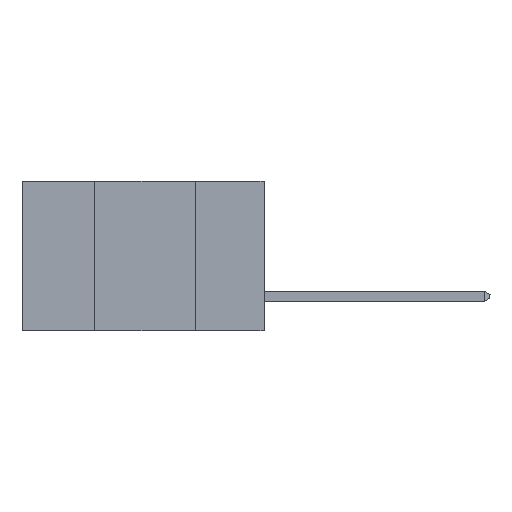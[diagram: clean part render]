
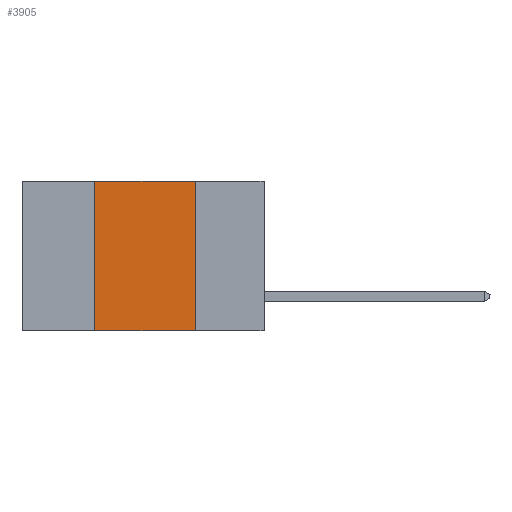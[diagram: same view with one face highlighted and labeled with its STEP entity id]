
A CAD part, left-side view. The second image highlights one B-rep face of the part: STEP entity #3905.
In plain terms, the highlighted planar face has unit normal (-1, 0, 0).
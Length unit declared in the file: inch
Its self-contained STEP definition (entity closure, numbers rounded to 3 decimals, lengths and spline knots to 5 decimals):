
#182 = LINE ( 'NONE', #5513, #4247 ) ;
#1077 = VECTOR ( 'NONE', #8774, 39.37008 ) ;
#1508 = EDGE_CURVE ( 'NONE', #16776, #15488, #14772, .T. ) ;
#1599 = CARTESIAN_POINT ( 'NONE',  ( 0., 0.17, -0.37 ) ) ;
#1852 = VERTEX_POINT ( 'NONE', #14670 ) ;
#2734 = VERTEX_POINT ( 'NONE', #1599 ) ;
#2995 = ORIENTED_EDGE ( 'NONE', *, *, #9193, .T. ) ;
#3342 = DIRECTION ( 'NONE',  ( 0., -1., 0. ) ) ;
#3349 = CARTESIAN_POINT ( 'NONE',  ( 0., 0.17, -0.37 ) ) ;
#3461 = LINE ( 'NONE', #15240, #1077 ) ;
#3570 = CARTESIAN_POINT ( 'NONE',  ( 0., 0.42, 0. ) ) ;
#3905 = ADVANCED_FACE ( 'NONE', ( #8144 ), #4037, .F. ) ;
#4037 = PLANE ( 'NONE',  #6929 ) ;
#4247 = VECTOR ( 'NONE', #15028, 39.37008 ) ;
#4609 = VECTOR ( 'NONE', #3342, 39.37008 ) ;
#4896 = ORIENTED_EDGE ( 'NONE', *, *, #5324, .F. ) ;
#4900 = ORIENTED_EDGE ( 'NONE', *, *, #1508, .F. ) ;
#4988 = EDGE_CURVE ( 'NONE', #1852, #16776, #3461, .T. ) ;
#5324 = EDGE_CURVE ( 'NONE', #15488, #2734, #6037, .T. ) ;
#5449 = EDGE_LOOP ( 'NONE', ( #4896, #4900, #12648, #2995 ) ) ;
#5513 = CARTESIAN_POINT ( 'NONE',  ( 0., 0.6, -0.37 ) ) ;
#6037 = LINE ( 'NONE', #3349, #12718 ) ;
#6929 = AXIS2_PLACEMENT_3D ( 'NONE', #9359, #14599, #8062 ) ;
#8062 = DIRECTION ( 'NONE',  ( 0., 0., -1. ) ) ;
#8144 = FACE_OUTER_BOUND ( 'NONE', #5449, .T. ) ;
#8774 = DIRECTION ( 'NONE',  ( 0., 0., 1. ) ) ;
#9193 = EDGE_CURVE ( 'NONE', #1852, #2734, #182, .T. ) ;
#9359 = CARTESIAN_POINT ( 'NONE',  ( 0., 0.6, 0. ) ) ;
#11323 = DIRECTION ( 'NONE',  ( 0., 0., -1. ) ) ;
#12648 = ORIENTED_EDGE ( 'NONE', *, *, #4988, .F. ) ;
#12718 = VECTOR ( 'NONE', #11323, 39.37008 ) ;
#14599 = DIRECTION ( 'NONE',  ( 1., 0., 0. ) ) ;
#14670 = CARTESIAN_POINT ( 'NONE',  ( 0., 0.42, -0.37 ) ) ;
#14772 = LINE ( 'NONE', #16242, #4609 ) ;
#15028 = DIRECTION ( 'NONE',  ( 0., -1., 0. ) ) ;
#15240 = CARTESIAN_POINT ( 'NONE',  ( 0., 0.42, -0.37 ) ) ;
#15488 = VERTEX_POINT ( 'NONE', #16904 ) ;
#16242 = CARTESIAN_POINT ( 'NONE',  ( 0., 0.6, 0. ) ) ;
#16776 = VERTEX_POINT ( 'NONE', #3570 ) ;
#16904 = CARTESIAN_POINT ( 'NONE',  ( 0., 0.17, 0. ) ) ;
